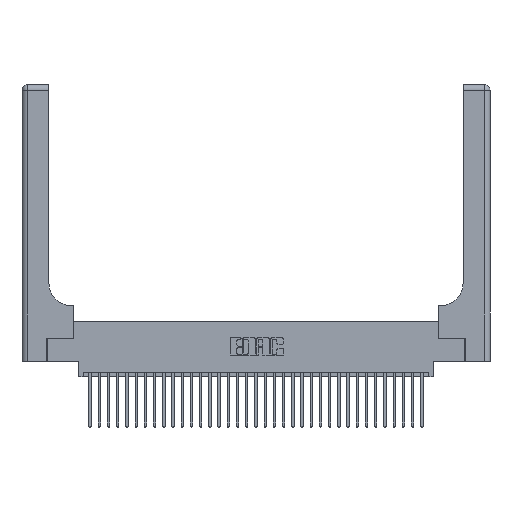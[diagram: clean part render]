
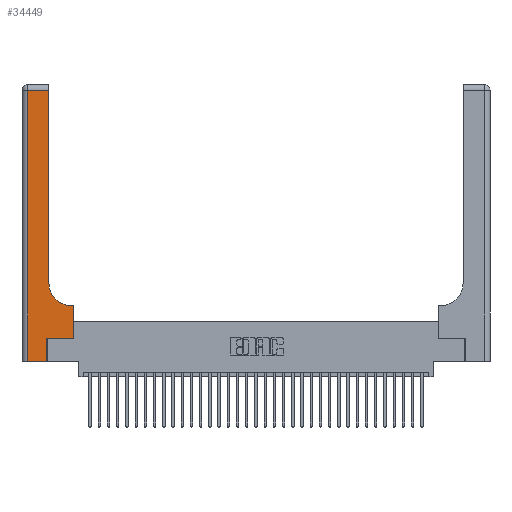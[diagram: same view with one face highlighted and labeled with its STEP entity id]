
A CAD part, top view. The second image highlights one B-rep face of the part: STEP entity #34449.
In plain terms, the highlighted planar face has unit normal (0, 0, 1).
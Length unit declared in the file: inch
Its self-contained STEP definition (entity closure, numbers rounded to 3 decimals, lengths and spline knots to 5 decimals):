
#336 = VERTEX_POINT ( 'NONE', #21079 ) ;
#1019 = DIRECTION ( 'NONE',  ( 1., 0., 0. ) ) ;
#1268 = EDGE_CURVE ( 'NONE', #22632, #336, #13835, .T. ) ;
#1764 = VERTEX_POINT ( 'NONE', #15688 ) ;
#2198 = CARTESIAN_POINT ( 'NONE',  ( 0.269, 0., 0.37 ) ) ;
#2743 = LINE ( 'NONE', #8323, #8255 ) ;
#3077 = EDGE_CURVE ( 'NONE', #7059, #1764, #2743, .T. ) ;
#3340 = LINE ( 'NONE', #12103, #24198 ) ;
#3827 = CARTESIAN_POINT ( 'NONE',  ( 0.06, 3., 0.37 ) ) ;
#3861 = CARTESIAN_POINT ( 'NONE',  ( 0.269, 0.25, 0.37 ) ) ;
#4816 = DIRECTION ( 'NONE',  ( 0., 0., -1. ) ) ;
#4961 = VECTOR ( 'NONE', #9159, 39.37008 ) ;
#5147 = DIRECTION ( 'NONE',  ( 0., 1., 0. ) ) ;
#5707 = DIRECTION ( 'NONE',  ( 0., 1., 0. ) ) ;
#7059 = VERTEX_POINT ( 'NONE', #27884 ) ;
#7919 = ORIENTED_EDGE ( 'NONE', *, *, #3077, .T. ) ;
#7981 = ORIENTED_EDGE ( 'NONE', *, *, #27614, .T. ) ;
#8255 = VECTOR ( 'NONE', #5707, 39.37008 ) ;
#8292 = DIRECTION ( 'NONE',  ( 0., 0., -1. ) ) ;
#8323 = CARTESIAN_POINT ( 'NONE',  ( 0.2915, 3., 0.37 ) ) ;
#8531 = VERTEX_POINT ( 'NONE', #13191 ) ;
#8893 = DIRECTION ( 'NONE',  ( 1., 0., 0. ) ) ;
#9159 = DIRECTION ( 'NONE',  ( 0., 1., 0. ) ) ;
#11683 = EDGE_CURVE ( 'NONE', #33179, #7059, #30651, .T. ) ;
#12068 = CARTESIAN_POINT ( 'NONE',  ( 0.269, 0., 0.37 ) ) ;
#12103 = CARTESIAN_POINT ( 'NONE',  ( 0., 2.94, 0.37 ) ) ;
#12443 = ORIENTED_EDGE ( 'NONE', *, *, #11683, .T. ) ;
#13191 = CARTESIAN_POINT ( 'NONE',  ( 0.06, 0., 0.37 ) ) ;
#13835 = LINE ( 'NONE', #19816, #4961 ) ;
#15397 = AXIS2_PLACEMENT_3D ( 'NONE', #26405, #4816, #26755 ) ;
#15408 = AXIS2_PLACEMENT_3D ( 'NONE', #16238, #8292, #30025 ) ;
#15580 = VECTOR ( 'NONE', #15594, 39.37008 ) ;
#15594 = DIRECTION ( 'NONE',  ( -1., 0., 0. ) ) ;
#15688 = CARTESIAN_POINT ( 'NONE',  ( 0.2915, 2.94, 0.37 ) ) ;
#16238 = CARTESIAN_POINT ( 'NONE',  ( 0., 3., 0.37 ) ) ;
#16792 = LINE ( 'NONE', #32774, #15580 ) ;
#19365 = VECTOR ( 'NONE', #8893, 39.37008 ) ;
#19631 = LINE ( 'NONE', #2198, #31986 ) ;
#19816 = CARTESIAN_POINT ( 'NONE',  ( 0.5585, 0.25, 0.37 ) ) ;
#19865 = EDGE_CURVE ( 'NONE', #336, #33179, #16792, .T. ) ;
#20276 = ORIENTED_EDGE ( 'NONE', *, *, #19865, .T. ) ;
#20586 = ORIENTED_EDGE ( 'NONE', *, *, #31034, .T. ) ;
#20631 = VERTEX_POINT ( 'NONE', #12068 ) ;
#21079 = CARTESIAN_POINT ( 'NONE',  ( 0.5585, 0.6, 0.37 ) ) ;
#21657 = CARTESIAN_POINT ( 'NONE',  ( 0.5415, 0.6, 0.37 ) ) ;
#21883 = CARTESIAN_POINT ( 'NONE',  ( 0.5585, 0.25, 0.37 ) ) ;
#22204 = VECTOR ( 'NONE', #1019, 39.37008 ) ;
#22325 = LINE ( 'NONE', #32972, #19365 ) ;
#22632 = VERTEX_POINT ( 'NONE', #21883 ) ;
#23392 = VECTOR ( 'NONE', #34071, 39.37008 ) ;
#23979 = ORIENTED_EDGE ( 'NONE', *, *, #31121, .T. ) ;
#24198 = VECTOR ( 'NONE', #25879, 39.37008 ) ;
#25339 = CARTESIAN_POINT ( 'NONE',  ( 0.269, 0.25, 0.37 ) ) ;
#25879 = DIRECTION ( 'NONE',  ( -1., 0., 0. ) ) ;
#26405 = CARTESIAN_POINT ( 'NONE',  ( 0.5415, 0.85, 0.37 ) ) ;
#26755 = DIRECTION ( 'NONE',  ( 1., 0., 0. ) ) ;
#26836 = PLANE ( 'NONE',  #15408 ) ;
#27333 = LINE ( 'NONE', #25339, #22204 ) ;
#27525 = ORIENTED_EDGE ( 'NONE', *, *, #1268, .T. ) ;
#27614 = EDGE_CURVE ( 'NONE', #20631, #28719, #19631, .T. ) ;
#27884 = CARTESIAN_POINT ( 'NONE',  ( 0.2915, 0.85, 0.37 ) ) ;
#28425 = ORIENTED_EDGE ( 'NONE', *, *, #31792, .T. ) ;
#28719 = VERTEX_POINT ( 'NONE', #3861 ) ;
#28900 = ORIENTED_EDGE ( 'NONE', *, *, #33448, .T. ) ;
#30016 = VERTEX_POINT ( 'NONE', #33880 ) ;
#30025 = DIRECTION ( 'NONE',  ( -1., 0., 0. ) ) ;
#30087 = EDGE_LOOP ( 'NONE', ( #7919, #23979, #28900, #20586, #7981, #28425, #27525, #20276, #12443 ) ) ;
#30562 = FACE_OUTER_BOUND ( 'NONE', #30087, .T. ) ;
#30651 = CIRCLE ( 'NONE', #15397, 0.25 ) ;
#31034 = EDGE_CURVE ( 'NONE', #8531, #20631, #22325, .T. ) ;
#31121 = EDGE_CURVE ( 'NONE', #1764, #30016, #3340, .T. ) ;
#31792 = EDGE_CURVE ( 'NONE', #28719, #22632, #27333, .T. ) ;
#31986 = VECTOR ( 'NONE', #5147, 39.37008 ) ;
#32297 = LINE ( 'NONE', #3827, #23392 ) ;
#32774 = CARTESIAN_POINT ( 'NONE',  ( 0.2915, 0.6, 0.37 ) ) ;
#32972 = CARTESIAN_POINT ( 'NONE',  ( 0., 0., 0.37 ) ) ;
#33179 = VERTEX_POINT ( 'NONE', #21657 ) ;
#33448 = EDGE_CURVE ( 'NONE', #30016, #8531, #32297, .T. ) ;
#33880 = CARTESIAN_POINT ( 'NONE',  ( 0.06, 2.94, 0.37 ) ) ;
#34071 = DIRECTION ( 'NONE',  ( 0., -1., 0. ) ) ;
#34449 = ADVANCED_FACE ( 'NONE', ( #30562 ), #26836, .F. ) ;
